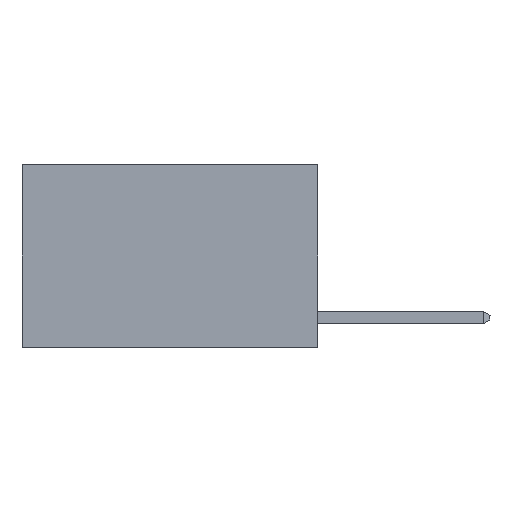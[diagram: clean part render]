
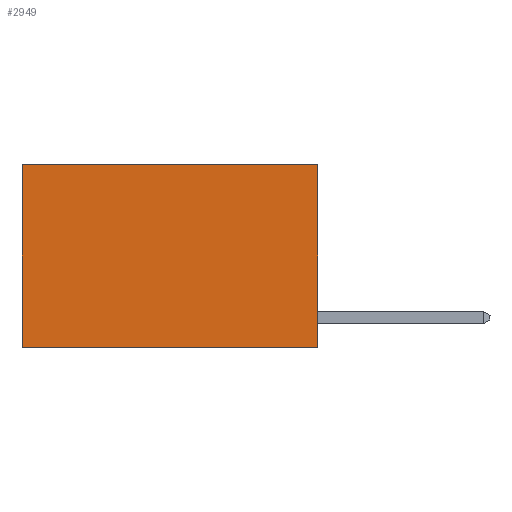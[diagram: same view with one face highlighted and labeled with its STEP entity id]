
A CAD part, left-side view. The second image highlights one B-rep face of the part: STEP entity #2949.
In plain terms, the highlighted planar face has unit normal (-1, 0, 0).
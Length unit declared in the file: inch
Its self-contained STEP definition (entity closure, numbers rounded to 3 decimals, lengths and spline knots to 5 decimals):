
#12 = CARTESIAN_POINT ( 'NONE',  ( 0.2625, 0., 0. ) ) ;
#236 = DIRECTION ( 'NONE',  ( 0., 0., -1. ) ) ;
#393 = EDGE_CURVE ( 'NONE', #5076, #8344, #5318, .T. ) ;
#461 = CARTESIAN_POINT ( 'NONE',  ( 0.2625, 0., 0. ) ) ;
#501 = LINE ( 'NONE', #7997, #5280 ) ;
#784 = DIRECTION ( 'NONE',  ( 0., 1., 0. ) ) ;
#1111 = VERTEX_POINT ( 'NONE', #7388 ) ;
#1656 = CARTESIAN_POINT ( 'NONE',  ( 0.2625, 0., -0.37 ) ) ;
#1661 = ORIENTED_EDGE ( 'NONE', *, *, #8053, .T. ) ;
#1805 = LINE ( 'NONE', #3856, #5970 ) ;
#2173 = EDGE_LOOP ( 'NONE', ( #1661, #3850, #7027, #5744 ) ) ;
#2429 = DIRECTION ( 'NONE',  ( 0., 0., -1. ) ) ;
#2557 = CARTESIAN_POINT ( 'NONE',  ( 0.2625, 0., 0. ) ) ;
#2949 = ADVANCED_FACE ( 'NONE', ( #7123 ), #7973, .F. ) ;
#3850 = ORIENTED_EDGE ( 'NONE', *, *, #8446, .F. ) ;
#3856 = CARTESIAN_POINT ( 'NONE',  ( 0.2625, 0.6, 0. ) ) ;
#4413 = CARTESIAN_POINT ( 'NONE',  ( 0.2625, 0.6, 0. ) ) ;
#5049 = DIRECTION ( 'NONE',  ( 0., 0., -1. ) ) ;
#5076 = VERTEX_POINT ( 'NONE', #2557 ) ;
#5141 = EDGE_CURVE ( 'NONE', #5076, #7164, #8455, .T. ) ;
#5280 = VECTOR ( 'NONE', #784, 39.37008 ) ;
#5318 = LINE ( 'NONE', #12, #6848 ) ;
#5744 = ORIENTED_EDGE ( 'NONE', *, *, #393, .T. ) ;
#5941 = DIRECTION ( 'NONE',  ( 1., 0., 0. ) ) ;
#5970 = VECTOR ( 'NONE', #5049, 39.37008 ) ;
#6309 = CARTESIAN_POINT ( 'NONE',  ( 0.2625, 0., 0. ) ) ;
#6346 = AXIS2_PLACEMENT_3D ( 'NONE', #461, #5941, #2429 ) ;
#6848 = VECTOR ( 'NONE', #8039, 39.37008 ) ;
#7027 = ORIENTED_EDGE ( 'NONE', *, *, #5141, .F. ) ;
#7123 = FACE_OUTER_BOUND ( 'NONE', #2173, .T. ) ;
#7164 = VERTEX_POINT ( 'NONE', #1656 ) ;
#7388 = CARTESIAN_POINT ( 'NONE',  ( 0.2625, 0.6, -0.37 ) ) ;
#7806 = VECTOR ( 'NONE', #236, 39.37008 ) ;
#7973 = PLANE ( 'NONE',  #6346 ) ;
#7997 = CARTESIAN_POINT ( 'NONE',  ( 0.2625, 0., -0.37 ) ) ;
#8039 = DIRECTION ( 'NONE',  ( 0., 1., 0. ) ) ;
#8053 = EDGE_CURVE ( 'NONE', #8344, #1111, #1805, .T. ) ;
#8344 = VERTEX_POINT ( 'NONE', #4413 ) ;
#8446 = EDGE_CURVE ( 'NONE', #7164, #1111, #501, .T. ) ;
#8455 = LINE ( 'NONE', #6309, #7806 ) ;
